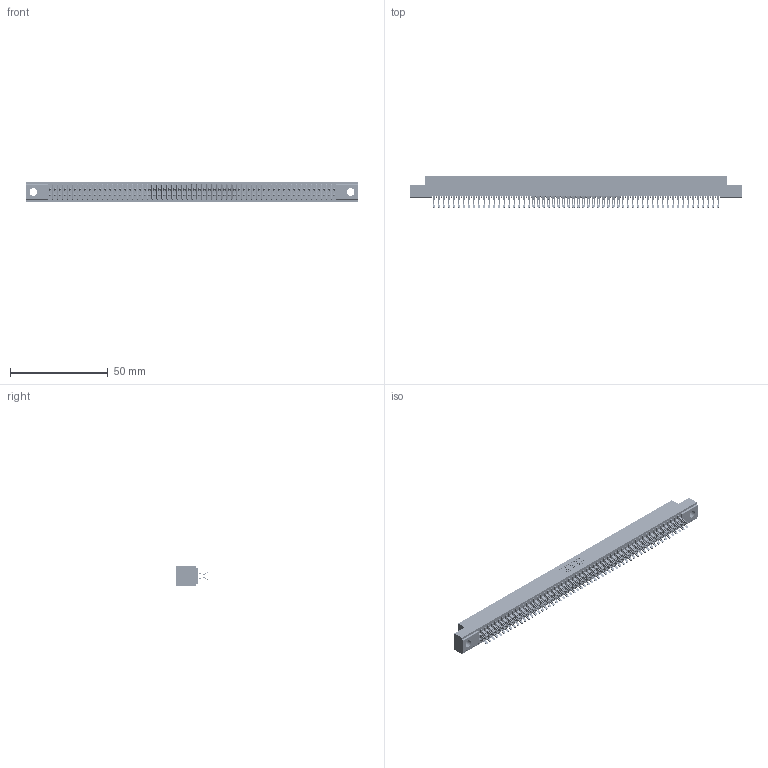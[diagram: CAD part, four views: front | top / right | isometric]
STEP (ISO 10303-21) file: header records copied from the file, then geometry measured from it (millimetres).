
FILE_DESCRIPTION (( 'STEP AP203' ), '1' );
FILE_NAME ('341-116-555-204.STEP', '2018-08-08T14:05:15', ( '' ), ( '' ), 'SwSTEP 2.0', 'SolidWorks 2016', '' );
FILE_SCHEMA (( 'CONFIG_CONTROL_DESIGN' ));
Length unit declared in the file: inch
Products named in the file (3): 341 Part_.156 (3.96) Dia Mounting Holes; 341-292-001_341-292-155; 341-116-555-204
Assembly tree (117 placements, depth 2):
  341-116-555-204
    341 Part_.156 (3.96) Dia Mounting Holes
    341-292-001_341-292-155  x116
Bounding box: 169.54 x 16.31 x 10.16 mm (x, y, z)
Volume: 12575.7 mm3; surface area: 23661.6 mm2
Topology: 117 solids, 117 shells, 9178 faces, 27438 edges, 17862 vertices
Faces by surface type: plane 4954, cylinder 3992, sphere 118, torus 114
Entity records: 68949 total; most frequent: CARTESIAN_POINT 11482, ORIENTED_EDGE 11400, DIRECTION 11114, EDGE_CURVE 5700, VECTOR 4614, LINE 4614, VERTEX_POINT 3602, AXIS2_PLACEMENT_3D 3250
